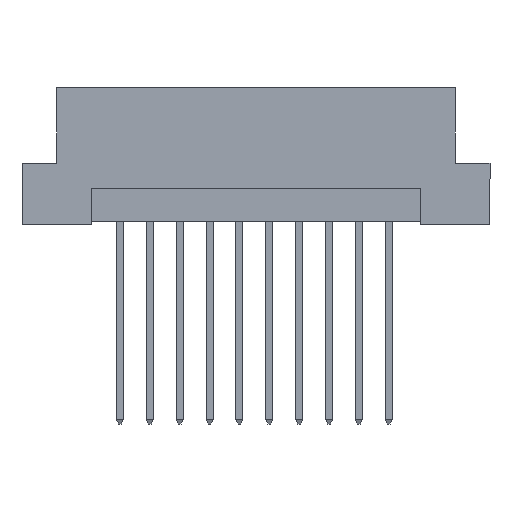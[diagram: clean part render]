
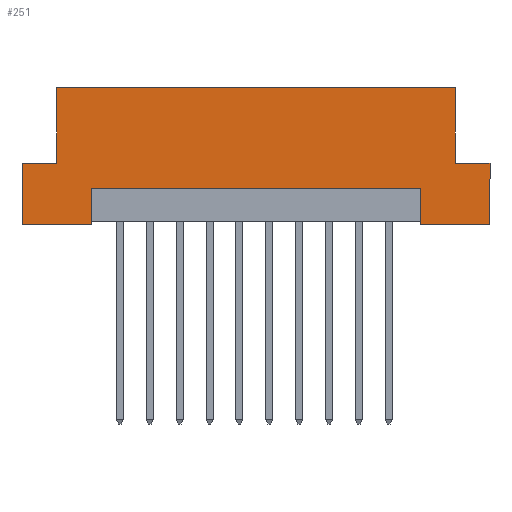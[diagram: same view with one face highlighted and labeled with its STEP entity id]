
A CAD part, front view. The second image highlights one B-rep face of the part: STEP entity #251.
In plain terms, the highlighted planar face has unit normal (0, -1, 0).
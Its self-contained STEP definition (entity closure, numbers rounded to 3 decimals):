
#114 = VERTEX_POINT ( 'NONE', #1781 ) ;
#141 = PLANE ( 'NONE',  #4255 ) ;
#151 = EDGE_CURVE ( 'NONE', #2951, #114, #1260, .T. ) ;
#210 = CARTESIAN_POINT ( 'NONE',  ( 16.94, -4.3, 5.2 ) ) ;
#212 = EDGE_CURVE ( 'NONE', #3546, #1607, #2317, .T. ) ;
#251 = ADVANCED_FACE ( 'NONE', ( #5187 ), #141, .F. ) ;
#266 = LINE ( 'NONE', #1124, #4541 ) ;
#276 = EDGE_CURVE ( 'NONE', #2425, #1370, #4029, .T. ) ;
#354 = EDGE_CURVE ( 'NONE', #1066, #4539, #972, .T. ) ;
#467 = CARTESIAN_POINT ( 'NONE',  ( -16.94, -4.3, 5.2 ) ) ;
#477 = ORIENTED_EDGE ( 'NONE', *, *, #1976, .T. ) ;
#491 = CARTESIAN_POINT ( 'NONE',  ( 16.94, -4.3, 5.2 ) ) ;
#493 = CARTESIAN_POINT ( 'NONE',  ( 19.9, -4.3, 5.2 ) ) ;
#561 = ORIENTED_EDGE ( 'NONE', *, *, #151, .F. ) ;
#623 = EDGE_CURVE ( 'NONE', #2951, #4539, #3073, .T. ) ;
#634 = DIRECTION ( 'NONE',  ( 1., 0., 0. ) ) ;
#776 = LINE ( 'NONE', #3299, #3991 ) ;
#865 = EDGE_CURVE ( 'NONE', #2404, #1607, #776, .T. ) ;
#939 = EDGE_CURVE ( 'NONE', #2425, #3311, #4158, .T. ) ;
#972 = LINE ( 'NONE', #1499, #1090 ) ;
#992 = LINE ( 'NONE', #3075, #4708 ) ;
#996 = VECTOR ( 'NONE', #2992, 1000. ) ;
#1028 = DIRECTION ( 'NONE',  ( 0., 1., 0. ) ) ;
#1066 = VERTEX_POINT ( 'NONE', #3599 ) ;
#1090 = VECTOR ( 'NONE', #1568, 1000. ) ;
#1124 = CARTESIAN_POINT ( 'NONE',  ( -14., -4.3, 0.2 ) ) ;
#1232 = ORIENTED_EDGE ( 'NONE', *, *, #1876, .F. ) ;
#1260 = LINE ( 'NONE', #493, #4973 ) ;
#1263 = LINE ( 'NONE', #467, #5304 ) ;
#1289 = EDGE_CURVE ( 'NONE', #3311, #2838, #992, .T. ) ;
#1370 = VERTEX_POINT ( 'NONE', #4407 ) ;
#1499 = CARTESIAN_POINT ( 'NONE',  ( 19.9, -4.3, 11.6 ) ) ;
#1568 = DIRECTION ( 'NONE',  ( 1., 0., 0. ) ) ;
#1607 = VERTEX_POINT ( 'NONE', #5076 ) ;
#1644 = EDGE_LOOP ( 'NONE', ( #4565, #4140, #477, #3082, #561, #3373, #4720, #4608, #1677, #5068, #4924, #1232 ) ) ;
#1677 = ORIENTED_EDGE ( 'NONE', *, *, #276, .F. ) ;
#1781 = CARTESIAN_POINT ( 'NONE',  ( 19.9, -4.3, 5.2 ) ) ;
#1857 = CARTESIAN_POINT ( 'NONE',  ( 19.9, -4.3, 0. ) ) ;
#1876 = EDGE_CURVE ( 'NONE', #3546, #2838, #266, .T. ) ;
#1976 = EDGE_CURVE ( 'NONE', #2404, #2354, #4649, .T. ) ;
#2261 = DIRECTION ( 'NONE',  ( -1., 0., 0. ) ) ;
#2305 = CARTESIAN_POINT ( 'NONE',  ( -14., -4.3, 3. ) ) ;
#2317 = LINE ( 'NONE', #4833, #3553 ) ;
#2321 = VECTOR ( 'NONE', #634, 1000. ) ;
#2354 = VERTEX_POINT ( 'NONE', #1857 ) ;
#2396 = CARTESIAN_POINT ( 'NONE',  ( -19.9, -4.3, 0. ) ) ;
#2404 = VERTEX_POINT ( 'NONE', #3154 ) ;
#2425 = VERTEX_POINT ( 'NONE', #4848 ) ;
#2801 = DIRECTION ( 'NONE',  ( 0., 0., -1. ) ) ;
#2838 = VERTEX_POINT ( 'NONE', #4361 ) ;
#2951 = VERTEX_POINT ( 'NONE', #491 ) ;
#2957 = DIRECTION ( 'NONE',  ( 0., 0., 1. ) ) ;
#2992 = DIRECTION ( 'NONE',  ( 0., 0., -1. ) ) ;
#3073 = LINE ( 'NONE', #210, #5137 ) ;
#3075 = CARTESIAN_POINT ( 'NONE',  ( 19.9, -4.3, 0. ) ) ;
#3079 = DIRECTION ( 'NONE',  ( 1., 0., 0. ) ) ;
#3082 = ORIENTED_EDGE ( 'NONE', *, *, #4288, .F. ) ;
#3095 = VECTOR ( 'NONE', #4113, 1000. ) ;
#3154 = CARTESIAN_POINT ( 'NONE',  ( 14., -4.3, 0. ) ) ;
#3250 = CARTESIAN_POINT ( 'NONE',  ( 19.9, -4.3, 11.6 ) ) ;
#3299 = CARTESIAN_POINT ( 'NONE',  ( 14., -4.3, 0.2 ) ) ;
#3311 = VERTEX_POINT ( 'NONE', #2396 ) ;
#3373 = ORIENTED_EDGE ( 'NONE', *, *, #623, .T. ) ;
#3438 = CARTESIAN_POINT ( 'NONE',  ( 19.9, -4.3, 0. ) ) ;
#3546 = VERTEX_POINT ( 'NONE', #2305 ) ;
#3553 = VECTOR ( 'NONE', #3079, 1000. ) ;
#3587 = DIRECTION ( 'NONE',  ( 0., 0., 1. ) ) ;
#3599 = CARTESIAN_POINT ( 'NONE',  ( -16.94, -4.3, 11.6 ) ) ;
#3651 = LINE ( 'NONE', #3250, #3095 ) ;
#3658 = CARTESIAN_POINT ( 'NONE',  ( 16.94, -4.3, 11.6 ) ) ;
#3804 = CARTESIAN_POINT ( 'NONE',  ( -19.9, -4.3, 11.6 ) ) ;
#3844 = VECTOR ( 'NONE', #4240, 1000. ) ;
#3885 = DIRECTION ( 'NONE',  ( 1., 0., 0. ) ) ;
#3991 = VECTOR ( 'NONE', #4996, 1000. ) ;
#4029 = LINE ( 'NONE', #4768, #2321 ) ;
#4113 = DIRECTION ( 'NONE',  ( 0., 0., -1. ) ) ;
#4140 = ORIENTED_EDGE ( 'NONE', *, *, #865, .F. ) ;
#4158 = LINE ( 'NONE', #3804, #996 ) ;
#4240 = DIRECTION ( 'NONE',  ( 1., 0., 0. ) ) ;
#4255 = AXIS2_PLACEMENT_3D ( 'NONE', #4326, #1028, #2261 ) ;
#4288 = EDGE_CURVE ( 'NONE', #114, #2354, #3651, .T. ) ;
#4326 = CARTESIAN_POINT ( 'NONE',  ( 19.9, -4.3, 11.6 ) ) ;
#4361 = CARTESIAN_POINT ( 'NONE',  ( -14., -4.3, 0. ) ) ;
#4407 = CARTESIAN_POINT ( 'NONE',  ( -16.94, -4.3, 5.2 ) ) ;
#4539 = VERTEX_POINT ( 'NONE', #3658 ) ;
#4541 = VECTOR ( 'NONE', #2801, 1000. ) ;
#4565 = ORIENTED_EDGE ( 'NONE', *, *, #212, .T. ) ;
#4608 = ORIENTED_EDGE ( 'NONE', *, *, #4643, .F. ) ;
#4643 = EDGE_CURVE ( 'NONE', #1370, #1066, #1263, .T. ) ;
#4649 = LINE ( 'NONE', #3438, #3844 ) ;
#4708 = VECTOR ( 'NONE', #3885, 1000. ) ;
#4720 = ORIENTED_EDGE ( 'NONE', *, *, #354, .F. ) ;
#4768 = CARTESIAN_POINT ( 'NONE',  ( -19.9, -4.3, 5.2 ) ) ;
#4833 = CARTESIAN_POINT ( 'NONE',  ( -14., -4.3, 3. ) ) ;
#4848 = CARTESIAN_POINT ( 'NONE',  ( -19.9, -4.3, 5.2 ) ) ;
#4924 = ORIENTED_EDGE ( 'NONE', *, *, #1289, .T. ) ;
#4973 = VECTOR ( 'NONE', #5165, 1000. ) ;
#4996 = DIRECTION ( 'NONE',  ( 0., 0., 1. ) ) ;
#5068 = ORIENTED_EDGE ( 'NONE', *, *, #939, .T. ) ;
#5076 = CARTESIAN_POINT ( 'NONE',  ( 14., -4.3, 3. ) ) ;
#5137 = VECTOR ( 'NONE', #3587, 1000. ) ;
#5165 = DIRECTION ( 'NONE',  ( 1., 0., 0. ) ) ;
#5187 = FACE_OUTER_BOUND ( 'NONE', #1644, .T. ) ;
#5304 = VECTOR ( 'NONE', #2957, 1000. ) ;
